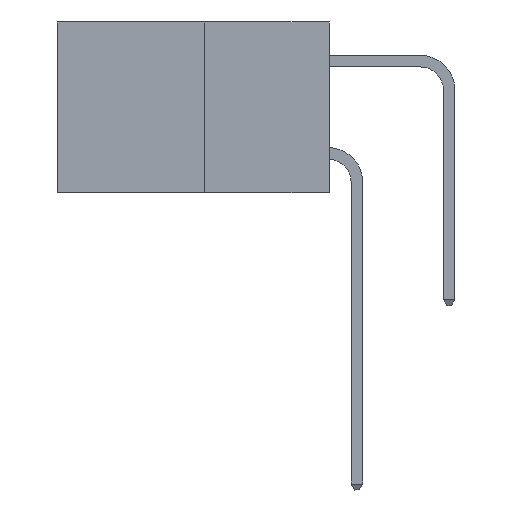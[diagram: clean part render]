
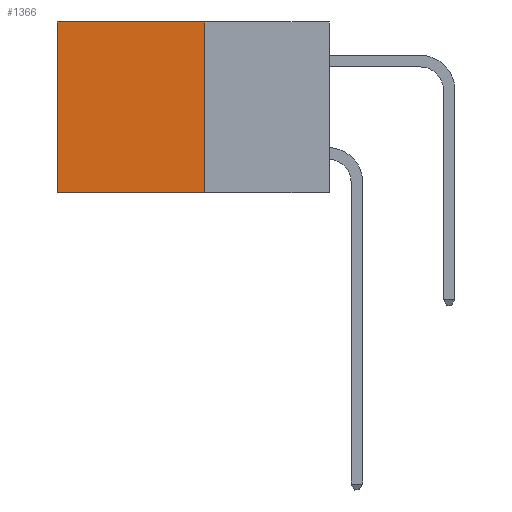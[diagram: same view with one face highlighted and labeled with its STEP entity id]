
A CAD part, left-side view. The second image highlights one B-rep face of the part: STEP entity #1366.
In plain terms, the highlighted planar face has unit normal (-1, 0, 0).
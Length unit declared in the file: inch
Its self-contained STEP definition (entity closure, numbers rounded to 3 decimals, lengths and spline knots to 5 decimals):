
#224 = CARTESIAN_POINT ( 'NONE',  ( 0.277, 0.27, 0. ) ) ;
#309 = DIRECTION ( 'NONE',  ( 0., 0., -1. ) ) ;
#400 = VERTEX_POINT ( 'NONE', #13070 ) ;
#474 = EDGE_CURVE ( 'NONE', #400, #8676, #9693, .T. ) ;
#493 = EDGE_CURVE ( 'NONE', #400, #10378, #9069, .T. ) ;
#696 = VECTOR ( 'NONE', #5476, 39.37008 ) ;
#844 = EDGE_CURVE ( 'NONE', #10378, #6340, #8756, .T. ) ;
#970 = ORIENTED_EDGE ( 'NONE', *, *, #474, .F. ) ;
#1366 = ADVANCED_FACE ( 'NONE', ( #3643 ), #7837, .F. ) ;
#1589 = DIRECTION ( 'NONE',  ( 0., 0., -1. ) ) ;
#1672 = CARTESIAN_POINT ( 'NONE',  ( 0.277, 0.27, -0.37 ) ) ;
#2011 = AXIS2_PLACEMENT_3D ( 'NONE', #1672, #8385, #1589 ) ;
#2568 = LINE ( 'NONE', #5914, #10411 ) ;
#2682 = CARTESIAN_POINT ( 'NONE',  ( 0.277, 0.59, 0. ) ) ;
#3261 = ORIENTED_EDGE ( 'NONE', *, *, #4653, .F. ) ;
#3643 = FACE_OUTER_BOUND ( 'NONE', #5833, .T. ) ;
#4653 = EDGE_CURVE ( 'NONE', #8676, #6340, #2568, .T. ) ;
#5017 = DIRECTION ( 'NONE',  ( 0., 0., -1. ) ) ;
#5476 = DIRECTION ( 'NONE',  ( 0., 1., 0. ) ) ;
#5833 = EDGE_LOOP ( 'NONE', ( #12371, #3261, #970, #9305 ) ) ;
#5914 = CARTESIAN_POINT ( 'NONE',  ( 0.277, 0.27, -0.37 ) ) ;
#6134 = VECTOR ( 'NONE', #309, 39.37008 ) ;
#6340 = VERTEX_POINT ( 'NONE', #8434 ) ;
#7048 = VECTOR ( 'NONE', #5017, 39.37008 ) ;
#7465 = CARTESIAN_POINT ( 'NONE',  ( 0.277, 0.59, -0.37 ) ) ;
#7837 = PLANE ( 'NONE',  #2011 ) ;
#8385 = DIRECTION ( 'NONE',  ( 1., 0., 0. ) ) ;
#8434 = CARTESIAN_POINT ( 'NONE',  ( 0.277, 0.59, -0.37 ) ) ;
#8676 = VERTEX_POINT ( 'NONE', #8811 ) ;
#8756 = LINE ( 'NONE', #7465, #6134 ) ;
#8811 = CARTESIAN_POINT ( 'NONE',  ( 0.277, 0.27, -0.37 ) ) ;
#9069 = LINE ( 'NONE', #224, #696 ) ;
#9305 = ORIENTED_EDGE ( 'NONE', *, *, #493, .T. ) ;
#9693 = LINE ( 'NONE', #11747, #7048 ) ;
#9958 = DIRECTION ( 'NONE',  ( 0., 1., 0. ) ) ;
#10378 = VERTEX_POINT ( 'NONE', #2682 ) ;
#10411 = VECTOR ( 'NONE', #9958, 39.37008 ) ;
#11747 = CARTESIAN_POINT ( 'NONE',  ( 0.277, 0.27, -0.37 ) ) ;
#12371 = ORIENTED_EDGE ( 'NONE', *, *, #844, .T. ) ;
#13070 = CARTESIAN_POINT ( 'NONE',  ( 0.277, 0.27, 0. ) ) ;
